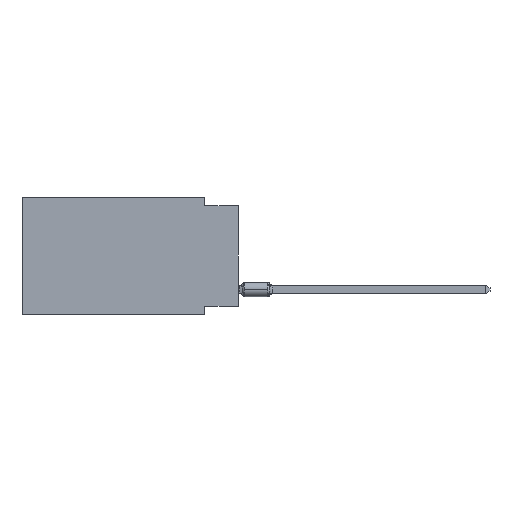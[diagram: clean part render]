
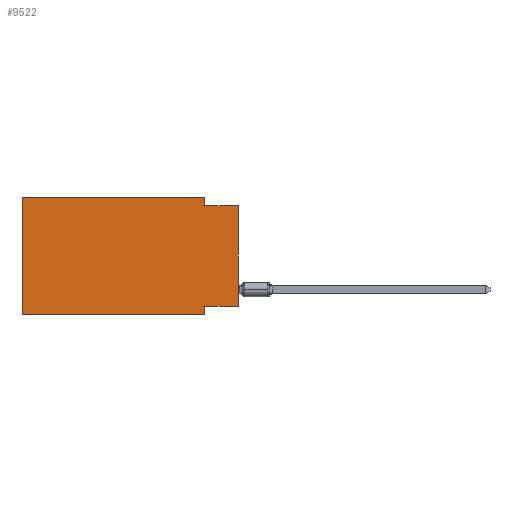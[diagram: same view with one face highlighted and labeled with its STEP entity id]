
A CAD part, left-side view. The second image highlights one B-rep face of the part: STEP entity #9522.
In plain terms, the highlighted planar face has unit normal (-1, 0, 0).
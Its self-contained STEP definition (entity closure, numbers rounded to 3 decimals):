
#261 = LINE ( 'NONE', #2525, #5480 ) ;
#317 = LINE ( 'NONE', #3041, #10584 ) ;
#323 = CARTESIAN_POINT ( 'NONE',  ( 0., 16.383, 0. ) ) ;
#464 = VERTEX_POINT ( 'NONE', #11613 ) ;
#1120 = DIRECTION ( 'NONE',  ( 0., 0., -1. ) ) ;
#1402 = AXIS2_PLACEMENT_3D ( 'NONE', #11249, #8605, #14454 ) ;
#1530 = CARTESIAN_POINT ( 'NONE',  ( 0., 16.383, 0. ) ) ;
#1687 = LINE ( 'NONE', #1530, #4572 ) ;
#2063 = EDGE_CURVE ( 'NONE', #4556, #4142, #2264, .T. ) ;
#2264 = LINE ( 'NONE', #11511, #7083 ) ;
#2270 = EDGE_CURVE ( 'NONE', #11109, #4142, #5306, .T. ) ;
#2525 = CARTESIAN_POINT ( 'NONE',  ( 0., 2.54, 0. ) ) ;
#2903 = DIRECTION ( 'NONE',  ( 0., 1., 0. ) ) ;
#3041 = CARTESIAN_POINT ( 'NONE',  ( 0., 0., -8.255 ) ) ;
#3604 = ORIENTED_EDGE ( 'NONE', *, *, #2063, .F. ) ;
#3791 = CARTESIAN_POINT ( 'NONE',  ( 0., 0., 0. ) ) ;
#3883 = VERTEX_POINT ( 'NONE', #323 ) ;
#4142 = VERTEX_POINT ( 'NONE', #13132 ) ;
#4436 = VERTEX_POINT ( 'NONE', #10295 ) ;
#4556 = VERTEX_POINT ( 'NONE', #14407 ) ;
#4572 = VECTOR ( 'NONE', #8451, 1000. ) ;
#4599 = EDGE_CURVE ( 'NONE', #3883, #9220, #6128, .T. ) ;
#5306 = LINE ( 'NONE', #10911, #13785 ) ;
#5404 = VERTEX_POINT ( 'NONE', #7439 ) ;
#5480 = VECTOR ( 'NONE', #6029, 1000. ) ;
#5812 = CARTESIAN_POINT ( 'NONE',  ( 0., 0., -0.635 ) ) ;
#6029 = DIRECTION ( 'NONE',  ( 0., 0., -1. ) ) ;
#6128 = LINE ( 'NONE', #10749, #11704 ) ;
#6666 = ORIENTED_EDGE ( 'NONE', *, *, #8724, .F. ) ;
#6701 = VECTOR ( 'NONE', #10537, 1000. ) ;
#7083 = VECTOR ( 'NONE', #1120, 1000. ) ;
#7434 = EDGE_LOOP ( 'NONE', ( #13331, #9010, #11209, #12072, #11988, #8214, #3604, #6666 ) ) ;
#7439 = CARTESIAN_POINT ( 'NONE',  ( 0., 2.54, -0.635 ) ) ;
#7552 = EDGE_CURVE ( 'NONE', #11109, #3883, #1687, .T. ) ;
#7720 = CARTESIAN_POINT ( 'NONE',  ( 0., 2.54, 0. ) ) ;
#8214 = ORIENTED_EDGE ( 'NONE', *, *, #2270, .T. ) ;
#8451 = DIRECTION ( 'NONE',  ( 0., 0., 1. ) ) ;
#8605 = DIRECTION ( 'NONE',  ( 1., 0., 0. ) ) ;
#8724 = EDGE_CURVE ( 'NONE', #464, #4556, #317, .T. ) ;
#9010 = ORIENTED_EDGE ( 'NONE', *, *, #9401, .F. ) ;
#9065 = LINE ( 'NONE', #5812, #9874 ) ;
#9220 = VERTEX_POINT ( 'NONE', #7720 ) ;
#9401 = EDGE_CURVE ( 'NONE', #5404, #4436, #9065, .T. ) ;
#9522 = ADVANCED_FACE ( 'NONE', ( #11107 ), #12097, .F. ) ;
#9657 = CARTESIAN_POINT ( 'NONE',  ( 0., 16.383, -8.89 ) ) ;
#9874 = VECTOR ( 'NONE', #13701, 1000. ) ;
#10295 = CARTESIAN_POINT ( 'NONE',  ( 0., 0., -0.635 ) ) ;
#10537 = DIRECTION ( 'NONE',  ( 0., 0., 1. ) ) ;
#10584 = VECTOR ( 'NONE', #2903, 1000. ) ;
#10683 = DIRECTION ( 'NONE',  ( 0., -1., 0. ) ) ;
#10749 = CARTESIAN_POINT ( 'NONE',  ( 0., 16.383, 0. ) ) ;
#10911 = CARTESIAN_POINT ( 'NONE',  ( 0., 16.383, -8.89 ) ) ;
#11107 = FACE_OUTER_BOUND ( 'NONE', #7434, .T. ) ;
#11109 = VERTEX_POINT ( 'NONE', #9657 ) ;
#11209 = ORIENTED_EDGE ( 'NONE', *, *, #13633, .F. ) ;
#11249 = CARTESIAN_POINT ( 'NONE',  ( 0., 16.383, 0. ) ) ;
#11435 = EDGE_CURVE ( 'NONE', #464, #4436, #14191, .T. ) ;
#11511 = CARTESIAN_POINT ( 'NONE',  ( 0., 2.54, -8.89 ) ) ;
#11613 = CARTESIAN_POINT ( 'NONE',  ( 0., 0., -8.255 ) ) ;
#11704 = VECTOR ( 'NONE', #10683, 1000. ) ;
#11988 = ORIENTED_EDGE ( 'NONE', *, *, #7552, .F. ) ;
#12072 = ORIENTED_EDGE ( 'NONE', *, *, #4599, .F. ) ;
#12097 = PLANE ( 'NONE',  #1402 ) ;
#13132 = CARTESIAN_POINT ( 'NONE',  ( 0., 2.54, -8.89 ) ) ;
#13331 = ORIENTED_EDGE ( 'NONE', *, *, #11435, .T. ) ;
#13416 = DIRECTION ( 'NONE',  ( 0., -1., 0. ) ) ;
#13633 = EDGE_CURVE ( 'NONE', #9220, #5404, #261, .T. ) ;
#13701 = DIRECTION ( 'NONE',  ( 0., -1., 0. ) ) ;
#13785 = VECTOR ( 'NONE', #13416, 1000. ) ;
#14191 = LINE ( 'NONE', #3791, #6701 ) ;
#14407 = CARTESIAN_POINT ( 'NONE',  ( 0., 2.54, -8.255 ) ) ;
#14454 = DIRECTION ( 'NONE',  ( 0., 0., -1. ) ) ;
